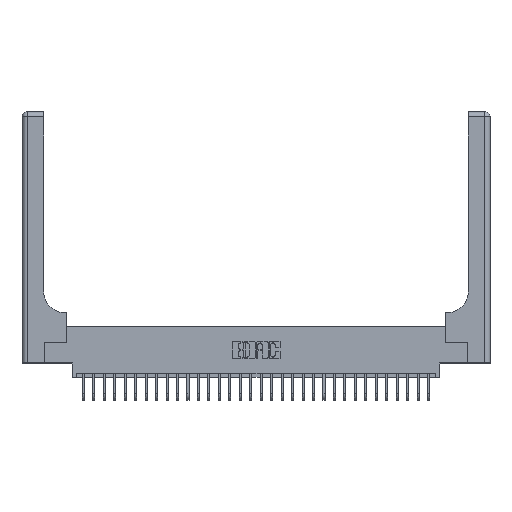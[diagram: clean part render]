
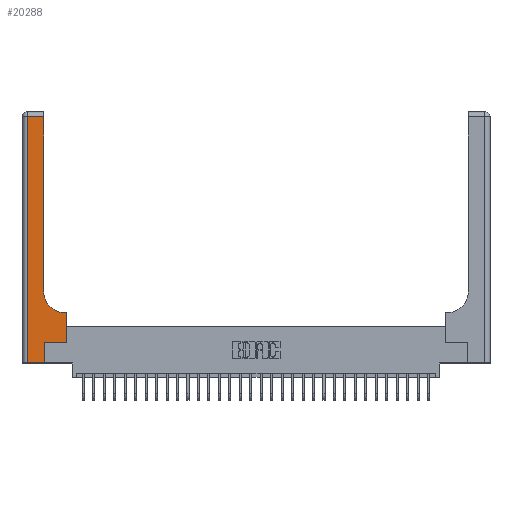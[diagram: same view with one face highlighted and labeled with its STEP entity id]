
A CAD part, top view. The second image highlights one B-rep face of the part: STEP entity #20288.
In plain terms, the highlighted planar face has unit normal (0, 0, 1).
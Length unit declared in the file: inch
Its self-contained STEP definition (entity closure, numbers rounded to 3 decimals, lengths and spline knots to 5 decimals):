
#159 = DIRECTION ( 'NONE',  ( -1., 0., 0. ) ) ;
#868 = VERTEX_POINT ( 'NONE', #11514 ) ;
#974 = ORIENTED_EDGE ( 'NONE', *, *, #24058, .T. ) ;
#1104 = CARTESIAN_POINT ( 'NONE',  ( 0.51, 0.85, 0.37 ) ) ;
#1549 = CARTESIAN_POINT ( 'NONE',  ( 0., 3., 0.37 ) ) ;
#1601 = VECTOR ( 'NONE', #2287, 39.37008 ) ;
#1864 = CARTESIAN_POINT ( 'NONE',  ( 0.265, 0., 0.37 ) ) ;
#2000 = DIRECTION ( 'NONE',  ( -1., 0., 0. ) ) ;
#2287 = DIRECTION ( 'NONE',  ( 0., -1., 0. ) ) ;
#2410 = EDGE_CURVE ( 'NONE', #11688, #22402, #8936, .T. ) ;
#2611 = CARTESIAN_POINT ( 'NONE',  ( 0.51, 0.6, 0.37 ) ) ;
#3091 = VECTOR ( 'NONE', #2000, 39.37008 ) ;
#3707 = CARTESIAN_POINT ( 'NONE',  ( 0., 2.94, 0.37 ) ) ;
#4193 = CARTESIAN_POINT ( 'NONE',  ( 0.528, 0.25, 0.37 ) ) ;
#5641 = ORIENTED_EDGE ( 'NONE', *, *, #19545, .T. ) ;
#5891 = EDGE_CURVE ( 'NONE', #13899, #27196, #27820, .T. ) ;
#6396 = CARTESIAN_POINT ( 'NONE',  ( 0.06, 3., 0.37 ) ) ;
#7625 = DIRECTION ( 'NONE',  ( -1., 0., 0. ) ) ;
#8020 = DIRECTION ( 'NONE',  ( 0., 1., 0. ) ) ;
#8188 = VECTOR ( 'NONE', #8020, 39.37008 ) ;
#8195 = CARTESIAN_POINT ( 'NONE',  ( 0.528, 0.6, 0.37 ) ) ;
#8383 = DIRECTION ( 'NONE',  ( 1., 0., 0. ) ) ;
#8844 = VERTEX_POINT ( 'NONE', #2611 ) ;
#8936 = LINE ( 'NONE', #15449, #26389 ) ;
#10849 = EDGE_CURVE ( 'NONE', #22505, #868, #16865, .T. ) ;
#10879 = ORIENTED_EDGE ( 'NONE', *, *, #26299, .T. ) ;
#11442 = VECTOR ( 'NONE', #159, 39.37008 ) ;
#11514 = CARTESIAN_POINT ( 'NONE',  ( 0.26, 2.94, 0.37 ) ) ;
#11688 = VERTEX_POINT ( 'NONE', #12503 ) ;
#12015 = FACE_OUTER_BOUND ( 'NONE', #14266, .T. ) ;
#12191 = DIRECTION ( 'NONE',  ( 0., 1., 0. ) ) ;
#12503 = CARTESIAN_POINT ( 'NONE',  ( 0.06, 0., 0.37 ) ) ;
#13183 = ORIENTED_EDGE ( 'NONE', *, *, #2410, .T. ) ;
#13899 = VERTEX_POINT ( 'NONE', #19536 ) ;
#13995 = VERTEX_POINT ( 'NONE', #18086 ) ;
#14168 = EDGE_CURVE ( 'NONE', #8844, #22505, #21345, .T. ) ;
#14265 = VECTOR ( 'NONE', #8383, 39.37008 ) ;
#14266 = EDGE_LOOP ( 'NONE', ( #25207, #20452, #10879, #13183, #21409, #21403, #5641, #974, #18162 ) ) ;
#14280 = PLANE ( 'NONE',  #25888 ) ;
#14735 = DIRECTION ( 'NONE',  ( 0., 1., 0. ) ) ;
#15149 = LINE ( 'NONE', #19699, #11442 ) ;
#15449 = CARTESIAN_POINT ( 'NONE',  ( 0., 0., 0.37 ) ) ;
#16806 = EDGE_CURVE ( 'NONE', #868, #13995, #21272, .T. ) ;
#16865 = LINE ( 'NONE', #27672, #25291 ) ;
#18038 = EDGE_CURVE ( 'NONE', #22402, #13899, #27527, .T. ) ;
#18086 = CARTESIAN_POINT ( 'NONE',  ( 0.06, 2.94, 0.37 ) ) ;
#18162 = ORIENTED_EDGE ( 'NONE', *, *, #14168, .T. ) ;
#18663 = DIRECTION ( 'NONE',  ( 0., 0., -1. ) ) ;
#18803 = DIRECTION ( 'NONE',  ( 1., 0., 0. ) ) ;
#19070 = AXIS2_PLACEMENT_3D ( 'NONE', #1104, #18663, #18803 ) ;
#19536 = CARTESIAN_POINT ( 'NONE',  ( 0.265, 0.25, 0.37 ) ) ;
#19545 = EDGE_CURVE ( 'NONE', #27196, #27010, #23631, .T. ) ;
#19603 = CARTESIAN_POINT ( 'NONE',  ( 0.265, 0., 0.37 ) ) ;
#19699 = CARTESIAN_POINT ( 'NONE',  ( 0.26, 0.6, 0.37 ) ) ;
#20288 = ADVANCED_FACE ( 'NONE', ( #12015 ), #14280, .F. ) ;
#20452 = ORIENTED_EDGE ( 'NONE', *, *, #16806, .T. ) ;
#21272 = LINE ( 'NONE', #3707, #3091 ) ;
#21345 = CIRCLE ( 'NONE', #19070, 0.25 ) ;
#21403 = ORIENTED_EDGE ( 'NONE', *, *, #5891, .T. ) ;
#21409 = ORIENTED_EDGE ( 'NONE', *, *, #18038, .T. ) ;
#22402 = VERTEX_POINT ( 'NONE', #19603 ) ;
#22505 = VERTEX_POINT ( 'NONE', #24987 ) ;
#23000 = CARTESIAN_POINT ( 'NONE',  ( 0.265, 0.25, 0.37 ) ) ;
#23631 = LINE ( 'NONE', #4193, #8188 ) ;
#24058 = EDGE_CURVE ( 'NONE', #27010, #8844, #15149, .T. ) ;
#24133 = DIRECTION ( 'NONE',  ( 1., 0., 0. ) ) ;
#24987 = CARTESIAN_POINT ( 'NONE',  ( 0.26, 0.85, 0.37 ) ) ;
#25207 = ORIENTED_EDGE ( 'NONE', *, *, #10849, .T. ) ;
#25291 = VECTOR ( 'NONE', #14735, 39.37008 ) ;
#25888 = AXIS2_PLACEMENT_3D ( 'NONE', #1549, #27072, #7625 ) ;
#26191 = CARTESIAN_POINT ( 'NONE',  ( 0.528, 0.25, 0.37 ) ) ;
#26299 = EDGE_CURVE ( 'NONE', #13995, #11688, #27686, .T. ) ;
#26389 = VECTOR ( 'NONE', #24133, 39.37008 ) ;
#26689 = VECTOR ( 'NONE', #12191, 39.37008 ) ;
#27010 = VERTEX_POINT ( 'NONE', #8195 ) ;
#27072 = DIRECTION ( 'NONE',  ( 0., 0., -1. ) ) ;
#27196 = VERTEX_POINT ( 'NONE', #26191 ) ;
#27527 = LINE ( 'NONE', #1864, #26689 ) ;
#27672 = CARTESIAN_POINT ( 'NONE',  ( 0.26, 3., 0.37 ) ) ;
#27686 = LINE ( 'NONE', #6396, #1601 ) ;
#27820 = LINE ( 'NONE', #23000, #14265 ) ;
